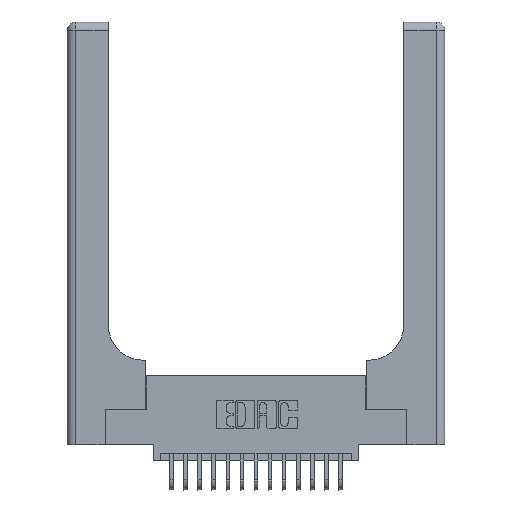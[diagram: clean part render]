
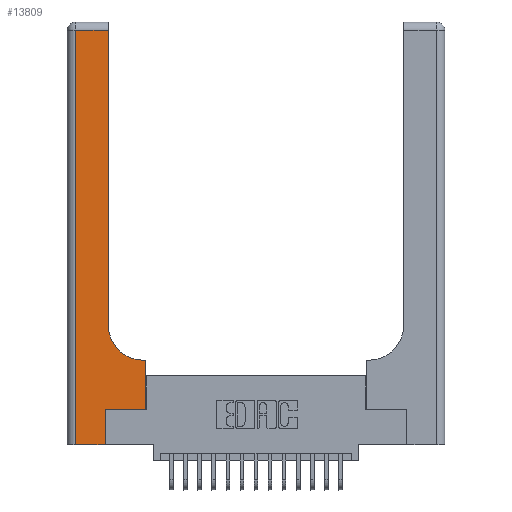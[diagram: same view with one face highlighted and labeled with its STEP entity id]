
A CAD part, top view. The second image highlights one B-rep face of the part: STEP entity #13809.
In plain terms, the highlighted planar face has unit normal (0, 0, 1).
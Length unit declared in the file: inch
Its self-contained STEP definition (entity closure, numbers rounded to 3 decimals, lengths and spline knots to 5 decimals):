
#241 = VERTEX_POINT ( 'NONE', #6239 ) ;
#814 = AXIS2_PLACEMENT_3D ( 'NONE', #17143, #15734, #15659 ) ;
#984 = CARTESIAN_POINT ( 'NONE',  ( 0.2915, 2.94, 0.37 ) ) ;
#1025 = DIRECTION ( 'NONE',  ( 1., 0., 0. ) ) ;
#1048 = VECTOR ( 'NONE', #7591, 39.37008 ) ;
#1128 = CARTESIAN_POINT ( 'NONE',  ( 0.06, 3., 0.37 ) ) ;
#1667 = ORIENTED_EDGE ( 'NONE', *, *, #15999, .T. ) ;
#1860 = CARTESIAN_POINT ( 'NONE',  ( 0.2915, 3., 0.37 ) ) ;
#2243 = ORIENTED_EDGE ( 'NONE', *, *, #5859, .T. ) ;
#2454 = LINE ( 'NONE', #1860, #4470 ) ;
#2593 = CARTESIAN_POINT ( 'NONE',  ( 0.269, 0., 0.37 ) ) ;
#2811 = EDGE_LOOP ( 'NONE', ( #18307, #16772, #3699, #2243, #19298, #18754, #1667, #15726, #14617 ) ) ;
#2967 = CARTESIAN_POINT ( 'NONE',  ( 0.269, 0., 0.37 ) ) ;
#3472 = DIRECTION ( 'NONE',  ( 0., 1., 0. ) ) ;
#3699 = ORIENTED_EDGE ( 'NONE', *, *, #12042, .T. ) ;
#3924 = VERTEX_POINT ( 'NONE', #15269 ) ;
#4056 = CARTESIAN_POINT ( 'NONE',  ( 0.5415, 0.6, 0.37 ) ) ;
#4233 = VECTOR ( 'NONE', #6033, 39.37008 ) ;
#4318 = VECTOR ( 'NONE', #19423, 39.37008 ) ;
#4470 = VECTOR ( 'NONE', #3472, 39.37008 ) ;
#4777 = VECTOR ( 'NONE', #21067, 39.37008 ) ;
#5016 = VERTEX_POINT ( 'NONE', #10525 ) ;
#5579 = CIRCLE ( 'NONE', #13661, 0.25 ) ;
#5615 = LINE ( 'NONE', #13086, #4318 ) ;
#5859 = EDGE_CURVE ( 'NONE', #13280, #12222, #12126, .T. ) ;
#5915 = PLANE ( 'NONE',  #814 ) ;
#6033 = DIRECTION ( 'NONE',  ( 0., -1., 0. ) ) ;
#6151 = EDGE_CURVE ( 'NONE', #241, #15542, #2454, .T. ) ;
#6239 = CARTESIAN_POINT ( 'NONE',  ( 0.2915, 0.85, 0.37 ) ) ;
#6507 = VECTOR ( 'NONE', #11698, 39.37008 ) ;
#6771 = EDGE_CURVE ( 'NONE', #17470, #9403, #13627, .T. ) ;
#7113 = CARTESIAN_POINT ( 'NONE',  ( 0.06, 0., 0.37 ) ) ;
#7591 = DIRECTION ( 'NONE',  ( 0., 1., 0. ) ) ;
#7985 = CARTESIAN_POINT ( 'NONE',  ( 0.2915, 0.6, 0.37 ) ) ;
#8614 = LINE ( 'NONE', #1128, #4233 ) ;
#9216 = EDGE_CURVE ( 'NONE', #5016, #14501, #10768, .T. ) ;
#9396 = DIRECTION ( 'NONE',  ( 0., 0., -1. ) ) ;
#9403 = VERTEX_POINT ( 'NONE', #14122 ) ;
#9726 = LINE ( 'NONE', #17237, #1048 ) ;
#10525 = CARTESIAN_POINT ( 'NONE',  ( 0.5585, 0.6, 0.37 ) ) ;
#10768 = LINE ( 'NONE', #7985, #14806 ) ;
#11165 = CARTESIAN_POINT ( 'NONE',  ( 0.5415, 0.85, 0.37 ) ) ;
#11320 = DIRECTION ( 'NONE',  ( -1., 0., 0. ) ) ;
#11698 = DIRECTION ( 'NONE',  ( 1., 0., 0. ) ) ;
#12042 = EDGE_CURVE ( 'NONE', #3924, #13280, #8614, .T. ) ;
#12126 = LINE ( 'NONE', #15395, #13404 ) ;
#12222 = VERTEX_POINT ( 'NONE', #2967 ) ;
#12678 = CARTESIAN_POINT ( 'NONE',  ( 0.269, 0.25, 0.37 ) ) ;
#13086 = CARTESIAN_POINT ( 'NONE',  ( 0., 2.94, 0.37 ) ) ;
#13280 = VERTEX_POINT ( 'NONE', #7113 ) ;
#13404 = VECTOR ( 'NONE', #1025, 39.37008 ) ;
#13627 = LINE ( 'NONE', #20918, #6507 ) ;
#13661 = AXIS2_PLACEMENT_3D ( 'NONE', #11165, #9396, #15926 ) ;
#13809 = ADVANCED_FACE ( 'NONE', ( #18699 ), #5915, .F. ) ;
#14122 = CARTESIAN_POINT ( 'NONE',  ( 0.5585, 0.25, 0.37 ) ) ;
#14501 = VERTEX_POINT ( 'NONE', #4056 ) ;
#14617 = ORIENTED_EDGE ( 'NONE', *, *, #18392, .T. ) ;
#14806 = VECTOR ( 'NONE', #11320, 39.37008 ) ;
#15269 = CARTESIAN_POINT ( 'NONE',  ( 0.06, 2.94, 0.37 ) ) ;
#15395 = CARTESIAN_POINT ( 'NONE',  ( 0., 0., 0.37 ) ) ;
#15542 = VERTEX_POINT ( 'NONE', #984 ) ;
#15659 = DIRECTION ( 'NONE',  ( -1., 0., 0. ) ) ;
#15726 = ORIENTED_EDGE ( 'NONE', *, *, #9216, .T. ) ;
#15734 = DIRECTION ( 'NONE',  ( 0., 0., -1. ) ) ;
#15926 = DIRECTION ( 'NONE',  ( 1., 0., 0. ) ) ;
#15999 = EDGE_CURVE ( 'NONE', #9403, #5016, #9726, .T. ) ;
#16371 = EDGE_CURVE ( 'NONE', #15542, #3924, #5615, .T. ) ;
#16772 = ORIENTED_EDGE ( 'NONE', *, *, #16371, .T. ) ;
#17143 = CARTESIAN_POINT ( 'NONE',  ( 0., 3., 0.37 ) ) ;
#17237 = CARTESIAN_POINT ( 'NONE',  ( 0.5585, 0.25, 0.37 ) ) ;
#17470 = VERTEX_POINT ( 'NONE', #12678 ) ;
#18307 = ORIENTED_EDGE ( 'NONE', *, *, #6151, .T. ) ;
#18392 = EDGE_CURVE ( 'NONE', #14501, #241, #5579, .T. ) ;
#18699 = FACE_OUTER_BOUND ( 'NONE', #2811, .T. ) ;
#18754 = ORIENTED_EDGE ( 'NONE', *, *, #6771, .T. ) ;
#18861 = EDGE_CURVE ( 'NONE', #12222, #17470, #19328, .T. ) ;
#19298 = ORIENTED_EDGE ( 'NONE', *, *, #18861, .T. ) ;
#19328 = LINE ( 'NONE', #2593, #4777 ) ;
#19423 = DIRECTION ( 'NONE',  ( -1., 0., 0. ) ) ;
#20918 = CARTESIAN_POINT ( 'NONE',  ( 0.269, 0.25, 0.37 ) ) ;
#21067 = DIRECTION ( 'NONE',  ( 0., 1., 0. ) ) ;
